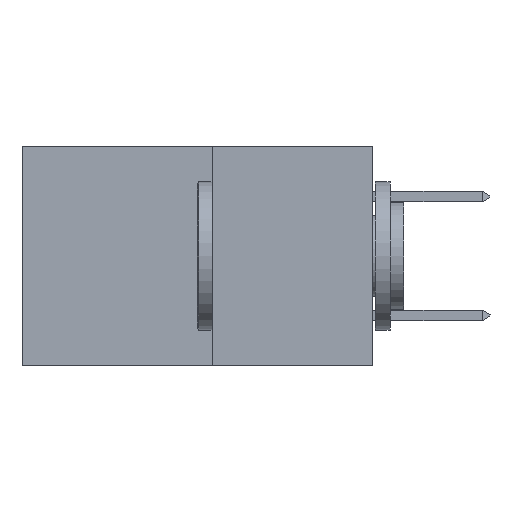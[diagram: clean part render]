
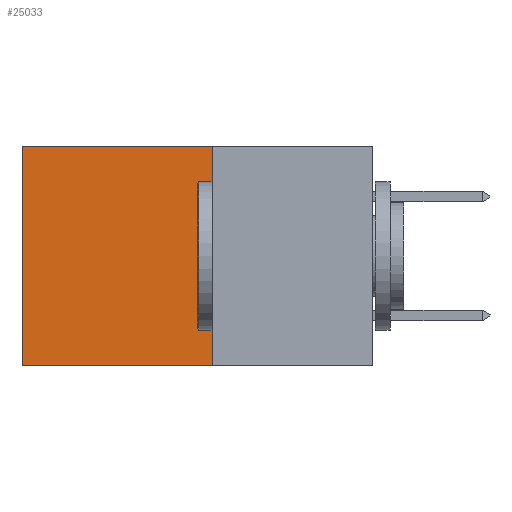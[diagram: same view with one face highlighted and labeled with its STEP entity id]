
A CAD part, left-side view. The second image highlights one B-rep face of the part: STEP entity #25033.
In plain terms, the highlighted planar face has unit normal (-1, 0, 0).
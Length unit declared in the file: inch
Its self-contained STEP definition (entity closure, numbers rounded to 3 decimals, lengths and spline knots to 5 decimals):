
#10 = ORIENTED_EDGE ( 'NONE', *, *, #78, .T. ) ;
#78 = EDGE_CURVE ( 'NONE', #6612, #11541, #23027, .T. ) ;
#548 = CARTESIAN_POINT ( 'NONE',  ( 0.277, 0.27, 0. ) ) ;
#2293 = EDGE_CURVE ( 'NONE', #21792, #16831, #23630, .T. ) ;
#3599 = CARTESIAN_POINT ( 'NONE',  ( 0.277, 0.27, -0.37 ) ) ;
#4040 = AXIS2_PLACEMENT_3D ( 'NONE', #5299, #26608, #9651 ) ;
#4921 = DIRECTION ( 'NONE',  ( 0., 0., -1. ) ) ;
#5299 = CARTESIAN_POINT ( 'NONE',  ( 0.277, 0.27, -0.37 ) ) ;
#5911 = VECTOR ( 'NONE', #11602, 39.37008 ) ;
#6158 = DIRECTION ( 'NONE',  ( 0., 1., 0. ) ) ;
#6367 = ORIENTED_EDGE ( 'NONE', *, *, #15935, .T. ) ;
#6524 = CARTESIAN_POINT ( 'NONE',  ( 0.277, 0.59, 0. ) ) ;
#6535 = VECTOR ( 'NONE', #6158, 39.37008 ) ;
#6612 = VERTEX_POINT ( 'NONE', #18193 ) ;
#7471 = PLANE ( 'NONE',  #4040 ) ;
#8972 = ORIENTED_EDGE ( 'NONE', *, *, #26561, .F. ) ;
#9610 = LINE ( 'NONE', #11457, #10968 ) ;
#9651 = DIRECTION ( 'NONE',  ( 0., 0., -1. ) ) ;
#10535 = CARTESIAN_POINT ( 'NONE',  ( 0.277, 0.27, -0.37 ) ) ;
#10968 = VECTOR ( 'NONE', #4921, 39.37008 ) ;
#11457 = CARTESIAN_POINT ( 'NONE',  ( 0.277, 0.59, -0.37 ) ) ;
#11541 = VERTEX_POINT ( 'NONE', #6524 ) ;
#11602 = DIRECTION ( 'NONE',  ( 0., 1., 0. ) ) ;
#11756 = EDGE_LOOP ( 'NONE', ( #6367, #21761, #8972, #10 ) ) ;
#12229 = DIRECTION ( 'NONE',  ( 0., 0., -1. ) ) ;
#13490 = LINE ( 'NONE', #3599, #24796 ) ;
#14212 = CARTESIAN_POINT ( 'NONE',  ( 0.277, 0.59, -0.37 ) ) ;
#15935 = EDGE_CURVE ( 'NONE', #11541, #16831, #9610, .T. ) ;
#16831 = VERTEX_POINT ( 'NONE', #14212 ) ;
#16899 = FACE_OUTER_BOUND ( 'NONE', #11756, .T. ) ;
#18193 = CARTESIAN_POINT ( 'NONE',  ( 0.277, 0.27, 0. ) ) ;
#21761 = ORIENTED_EDGE ( 'NONE', *, *, #2293, .F. ) ;
#21792 = VERTEX_POINT ( 'NONE', #23140 ) ;
#23027 = LINE ( 'NONE', #548, #5911 ) ;
#23140 = CARTESIAN_POINT ( 'NONE',  ( 0.277, 0.27, -0.37 ) ) ;
#23630 = LINE ( 'NONE', #10535, #6535 ) ;
#24796 = VECTOR ( 'NONE', #12229, 39.37008 ) ;
#25033 = ADVANCED_FACE ( 'NONE', ( #16899 ), #7471, .F. ) ;
#26561 = EDGE_CURVE ( 'NONE', #6612, #21792, #13490, .T. ) ;
#26608 = DIRECTION ( 'NONE',  ( 1., 0., 0. ) ) ;
